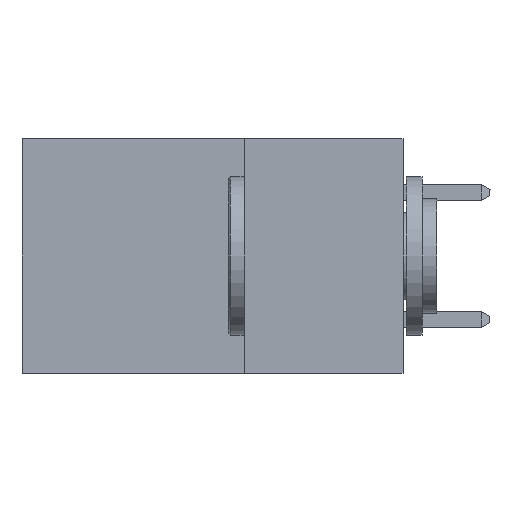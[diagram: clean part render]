
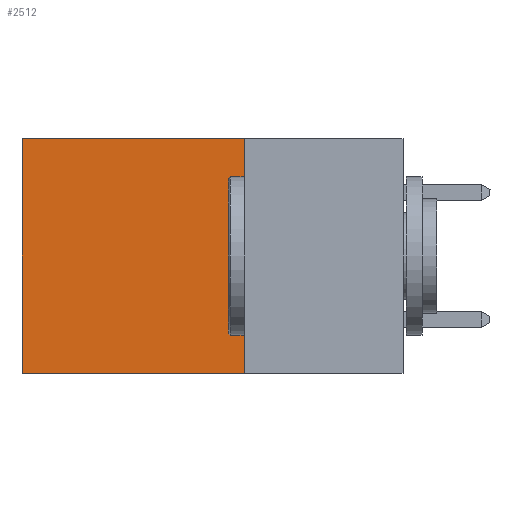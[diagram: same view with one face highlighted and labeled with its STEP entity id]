
A CAD part, left-side view. The second image highlights one B-rep face of the part: STEP entity #2512.
In plain terms, the highlighted planar face has unit normal (-1, 0, 0).
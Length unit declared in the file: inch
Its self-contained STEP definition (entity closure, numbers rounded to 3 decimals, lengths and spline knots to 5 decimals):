
#1013 = ORIENTED_EDGE ( 'NONE', *, *, #28642, .T. ) ;
#2512 = ADVANCED_FACE ( 'NONE', ( #24870 ), #28087, .F. ) ;
#2586 = CARTESIAN_POINT ( 'NONE',  ( 0.2875, 0.6, 0. ) ) ;
#4545 = AXIS2_PLACEMENT_3D ( 'NONE', #6411, #38902, #17365 ) ;
#6411 = CARTESIAN_POINT ( 'NONE',  ( 0.2875, 0.25, 0. ) ) ;
#6707 = ORIENTED_EDGE ( 'NONE', *, *, #21820, .F. ) ;
#8080 = LINE ( 'NONE', #43030, #45214 ) ;
#8826 = LINE ( 'NONE', #40738, #45943 ) ;
#9481 = VERTEX_POINT ( 'NONE', #2586 ) ;
#10379 = LINE ( 'NONE', #22563, #37999 ) ;
#14425 = EDGE_LOOP ( 'NONE', ( #28612, #40482, #6707, #1013 ) ) ;
#14462 = DIRECTION ( 'NONE',  ( 0., 1., 0. ) ) ;
#15594 = DIRECTION ( 'NONE',  ( 0., 1., 0. ) ) ;
#17365 = DIRECTION ( 'NONE',  ( 0., 0., -1. ) ) ;
#19500 = VERTEX_POINT ( 'NONE', #39022 ) ;
#21820 = EDGE_CURVE ( 'NONE', #42164, #19500, #22013, .T. ) ;
#22013 = LINE ( 'NONE', #35699, #34939 ) ;
#22563 = CARTESIAN_POINT ( 'NONE',  ( 0.2875, 0.6, 0. ) ) ;
#24870 = FACE_OUTER_BOUND ( 'NONE', #14425, .T. ) ;
#25191 = CARTESIAN_POINT ( 'NONE',  ( 0.2875, 0.6, -0.37 ) ) ;
#26151 = DIRECTION ( 'NONE',  ( 0., 0., -1. ) ) ;
#28087 = PLANE ( 'NONE',  #4545 ) ;
#28612 = ORIENTED_EDGE ( 'NONE', *, *, #44161, .T. ) ;
#28642 = EDGE_CURVE ( 'NONE', #42164, #9481, #8080, .T. ) ;
#34939 = VECTOR ( 'NONE', #39283, 39.37008 ) ;
#34998 = EDGE_CURVE ( 'NONE', #19500, #37226, #8826, .T. ) ;
#35699 = CARTESIAN_POINT ( 'NONE',  ( 0.2875, 0.25, 0. ) ) ;
#37226 = VERTEX_POINT ( 'NONE', #25191 ) ;
#37999 = VECTOR ( 'NONE', #26151, 39.37008 ) ;
#38902 = DIRECTION ( 'NONE',  ( 1., 0., 0. ) ) ;
#39022 = CARTESIAN_POINT ( 'NONE',  ( 0.2875, 0.25, -0.37 ) ) ;
#39283 = DIRECTION ( 'NONE',  ( 0., 0., -1. ) ) ;
#40482 = ORIENTED_EDGE ( 'NONE', *, *, #34998, .F. ) ;
#40738 = CARTESIAN_POINT ( 'NONE',  ( 0.2875, 0.25, -0.37 ) ) ;
#42164 = VERTEX_POINT ( 'NONE', #44494 ) ;
#43030 = CARTESIAN_POINT ( 'NONE',  ( 0.2875, 0.25, 0. ) ) ;
#44161 = EDGE_CURVE ( 'NONE', #9481, #37226, #10379, .T. ) ;
#44494 = CARTESIAN_POINT ( 'NONE',  ( 0.2875, 0.25, 0. ) ) ;
#45214 = VECTOR ( 'NONE', #14462, 39.37008 ) ;
#45943 = VECTOR ( 'NONE', #15594, 39.37008 ) ;
